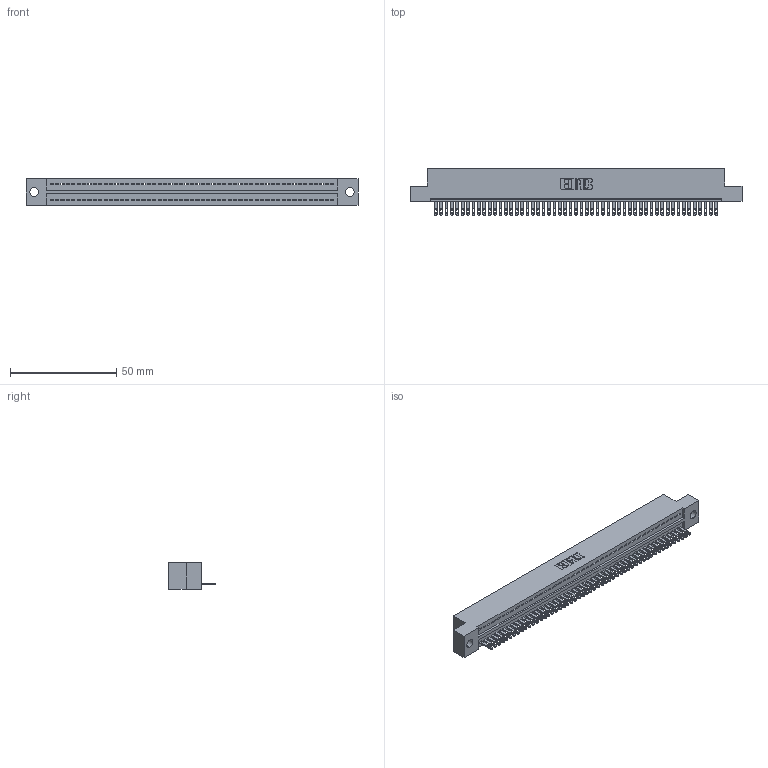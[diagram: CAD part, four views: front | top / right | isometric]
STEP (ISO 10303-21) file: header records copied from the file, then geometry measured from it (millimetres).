
FILE_DESCRIPTION (( 'STEP AP203' ), '1' );
FILE_NAME ('325-053-500-109.STEP', '2020-02-25T00:37:51', ( '' ), ( '' ), 'SwSTEP 2.0', 'SolidWorks 2016', '' );
FILE_SCHEMA (( 'CONFIG_CONTROL_DESIGN' ));
Length unit declared in the file: inch
Products named in the file (3): 325 Part_.160 TH; 325-292-001_325-293-100; 325-053-500-109
Assembly tree (54 placements, depth 2):
  325-053-500-109
    325 Part_.160 TH
    325-292-001_325-293-100  x53
Bounding box: 156.34 x 21.84 x 12.45 mm (x, y, z)
Volume: 19735.6 mm3; surface area: 21767.6 mm2
Topology: 54 solids, 54 shells, 2976 faces, 9215 edges, 6142 vertices
Faces by surface type: plane 1978, cylinder 998
Entity records: 30911 total; most frequent: CARTESIAN_POINT 5337, ORIENTED_EDGE 5326, DIRECTION 4481, EDGE_CURVE 2663, VECTOR 2531, LINE 2531, VERTEX_POINT 1774, AXIS2_PLACEMENT_3D 975
